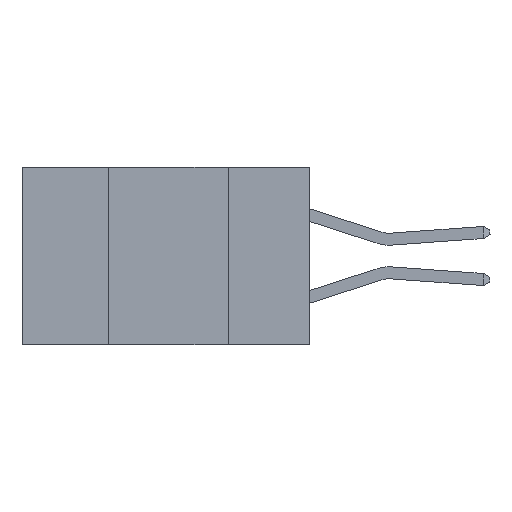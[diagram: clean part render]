
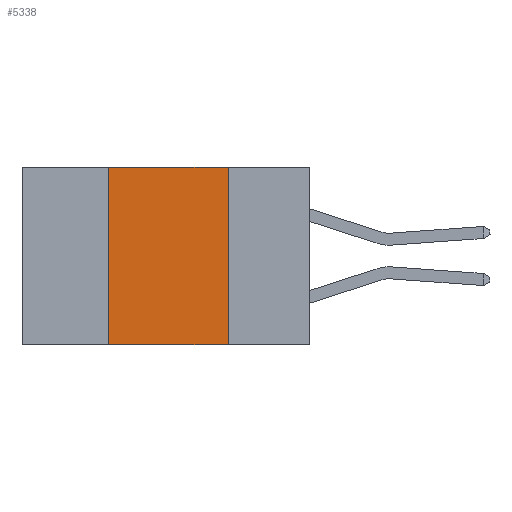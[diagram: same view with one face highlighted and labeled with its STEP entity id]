
A CAD part, left-side view. The second image highlights one B-rep face of the part: STEP entity #5338.
In plain terms, the highlighted planar face has unit normal (-1, 0, 0).
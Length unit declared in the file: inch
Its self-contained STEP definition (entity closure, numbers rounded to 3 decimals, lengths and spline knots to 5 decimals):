
#65 = CARTESIAN_POINT ( 'NONE',  ( 0., 0.17, 0. ) ) ;
#299 = VERTEX_POINT ( 'NONE', #65 ) ;
#672 = CARTESIAN_POINT ( 'NONE',  ( 0., 0.6, -0.37 ) ) ;
#704 = ORIENTED_EDGE ( 'NONE', *, *, #7799, .F. ) ;
#860 = CARTESIAN_POINT ( 'NONE',  ( 0., 0.17, -0.37 ) ) ;
#1999 = PLANE ( 'NONE',  #4894 ) ;
#2053 = VECTOR ( 'NONE', #5871, 39.37008 ) ;
#2699 = CARTESIAN_POINT ( 'NONE',  ( 0., 0.6, 0. ) ) ;
#2804 = VECTOR ( 'NONE', #6737, 39.37008 ) ;
#2812 = CARTESIAN_POINT ( 'NONE',  ( 0., 0.17, -0.37 ) ) ;
#2860 = LINE ( 'NONE', #2812, #2053 ) ;
#3061 = CARTESIAN_POINT ( 'NONE',  ( 0., 0.42, -0.37 ) ) ;
#3402 = DIRECTION ( 'NONE',  ( 0., 0., -1. ) ) ;
#3617 = LINE ( 'NONE', #672, #5733 ) ;
#4055 = EDGE_CURVE ( 'NONE', #5730, #299, #4917, .T. ) ;
#4894 = AXIS2_PLACEMENT_3D ( 'NONE', #7125, #7080, #3402 ) ;
#4917 = LINE ( 'NONE', #2699, #6598 ) ;
#5338 = ADVANCED_FACE ( 'NONE', ( #9395 ), #1999, .F. ) ;
#5685 = ORIENTED_EDGE ( 'NONE', *, *, #4055, .F. ) ;
#5730 = VERTEX_POINT ( 'NONE', #5821 ) ;
#5733 = VECTOR ( 'NONE', #6710, 39.37008 ) ;
#5821 = CARTESIAN_POINT ( 'NONE',  ( 0., 0.42, 0. ) ) ;
#5871 = DIRECTION ( 'NONE',  ( 0., 0., -1. ) ) ;
#6526 = VERTEX_POINT ( 'NONE', #860 ) ;
#6529 = VERTEX_POINT ( 'NONE', #3061 ) ;
#6598 = VECTOR ( 'NONE', #8897, 39.37008 ) ;
#6678 = ORIENTED_EDGE ( 'NONE', *, *, #7410, .F. ) ;
#6710 = DIRECTION ( 'NONE',  ( 0., -1., 0. ) ) ;
#6737 = DIRECTION ( 'NONE',  ( 0., 0., 1. ) ) ;
#7080 = DIRECTION ( 'NONE',  ( 1., 0., 0. ) ) ;
#7125 = CARTESIAN_POINT ( 'NONE',  ( 0., 0.6, 0. ) ) ;
#7410 = EDGE_CURVE ( 'NONE', #6529, #5730, #9784, .T. ) ;
#7507 = CARTESIAN_POINT ( 'NONE',  ( 0., 0.42, -0.37 ) ) ;
#7743 = EDGE_CURVE ( 'NONE', #6529, #6526, #3617, .T. ) ;
#7799 = EDGE_CURVE ( 'NONE', #299, #6526, #2860, .T. ) ;
#8656 = EDGE_LOOP ( 'NONE', ( #704, #5685, #6678, #8930 ) ) ;
#8897 = DIRECTION ( 'NONE',  ( 0., -1., 0. ) ) ;
#8930 = ORIENTED_EDGE ( 'NONE', *, *, #7743, .T. ) ;
#9395 = FACE_OUTER_BOUND ( 'NONE', #8656, .T. ) ;
#9784 = LINE ( 'NONE', #7507, #2804 ) ;
